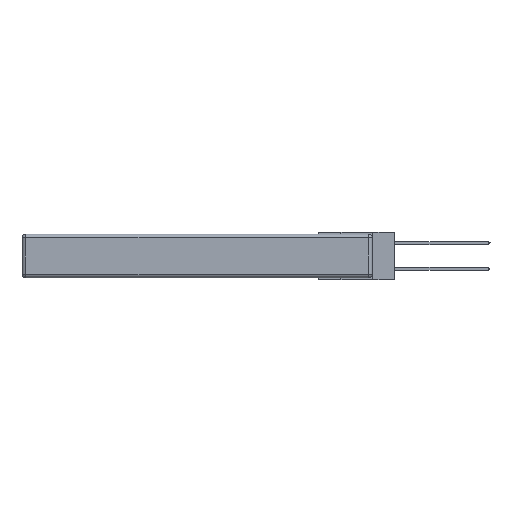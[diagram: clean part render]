
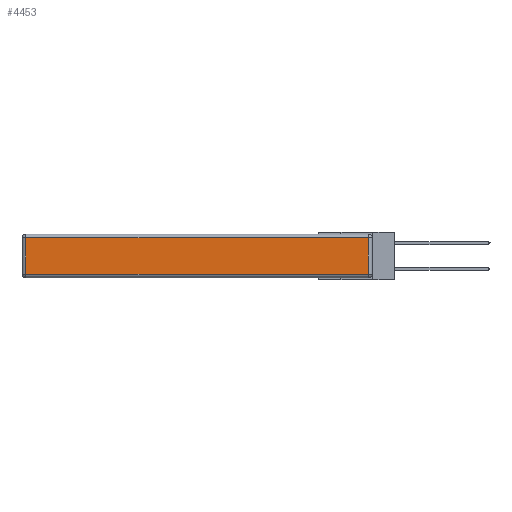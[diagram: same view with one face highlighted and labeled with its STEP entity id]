
A CAD part, left-side view. The second image highlights one B-rep face of the part: STEP entity #4453.
In plain terms, the highlighted planar face has unit normal (-1, 0, 0).
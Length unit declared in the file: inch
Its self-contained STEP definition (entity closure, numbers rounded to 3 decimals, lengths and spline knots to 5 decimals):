
#53 = CARTESIAN_POINT ( 'NONE',  ( 0., 0., -0.343 ) ) ;
#372 = ORIENTED_EDGE ( 'NONE', *, *, #7467, .T. ) ;
#662 = ORIENTED_EDGE ( 'NONE', *, *, #6120, .T. ) ;
#1039 = CARTESIAN_POINT ( 'NONE',  ( 0., 0.03, -0.03 ) ) ;
#1231 = VERTEX_POINT ( 'NONE', #1039 ) ;
#2381 = LINE ( 'NONE', #11488, #6825 ) ;
#2660 = CARTESIAN_POINT ( 'NONE',  ( 0., 2.72, -0.03 ) ) ;
#2822 = VERTEX_POINT ( 'NONE', #10932 ) ;
#3102 = DIRECTION ( 'NONE',  ( 0., -1., 0. ) ) ;
#3299 = PLANE ( 'NONE',  #6303 ) ;
#3773 = DIRECTION ( 'NONE',  ( 0., 1., 0. ) ) ;
#4119 = EDGE_CURVE ( 'NONE', #5745, #1231, #12724, .T. ) ;
#4453 = ADVANCED_FACE ( 'NONE', ( #7239 ), #3299, .T. ) ;
#5538 = CARTESIAN_POINT ( 'NONE',  ( 0., 0.03, -0.313 ) ) ;
#5745 = VERTEX_POINT ( 'NONE', #5538 ) ;
#5814 = DIRECTION ( 'NONE',  ( 0., 0., 1. ) ) ;
#6120 = EDGE_CURVE ( 'NONE', #2822, #5745, #2381, .T. ) ;
#6303 = AXIS2_PLACEMENT_3D ( 'NONE', #53, #7712, #10971 ) ;
#6825 = VECTOR ( 'NONE', #3102, 39.37008 ) ;
#6952 = VECTOR ( 'NONE', #3773, 39.37008 ) ;
#6965 = CARTESIAN_POINT ( 'NONE',  ( 0., 2.75, -0.03 ) ) ;
#7239 = FACE_OUTER_BOUND ( 'NONE', #13760, .T. ) ;
#7467 = EDGE_CURVE ( 'NONE', #9126, #2822, #13045, .T. ) ;
#7498 = LINE ( 'NONE', #6965, #6952 ) ;
#7712 = DIRECTION ( 'NONE',  ( -1., 0., 0. ) ) ;
#7918 = CARTESIAN_POINT ( 'NONE',  ( 0., 0.03, -0.343 ) ) ;
#8607 = ORIENTED_EDGE ( 'NONE', *, *, #4119, .T. ) ;
#9126 = VERTEX_POINT ( 'NONE', #2660 ) ;
#10049 = DIRECTION ( 'NONE',  ( 0., 0., -1. ) ) ;
#10300 = VECTOR ( 'NONE', #10049, 39.37008 ) ;
#10932 = CARTESIAN_POINT ( 'NONE',  ( 0., 2.72, -0.313 ) ) ;
#10971 = DIRECTION ( 'NONE',  ( 0., 0., 1. ) ) ;
#11488 = CARTESIAN_POINT ( 'NONE',  ( 0., 0., -0.313 ) ) ;
#11708 = VECTOR ( 'NONE', #5814, 39.37008 ) ;
#12224 = ORIENTED_EDGE ( 'NONE', *, *, #13162, .T. ) ;
#12724 = LINE ( 'NONE', #7918, #11708 ) ;
#13045 = LINE ( 'NONE', #13140, #10300 ) ;
#13140 = CARTESIAN_POINT ( 'NONE',  ( 0., 2.72, -0.343 ) ) ;
#13162 = EDGE_CURVE ( 'NONE', #1231, #9126, #7498, .T. ) ;
#13760 = EDGE_LOOP ( 'NONE', ( #662, #8607, #12224, #372 ) ) ;
